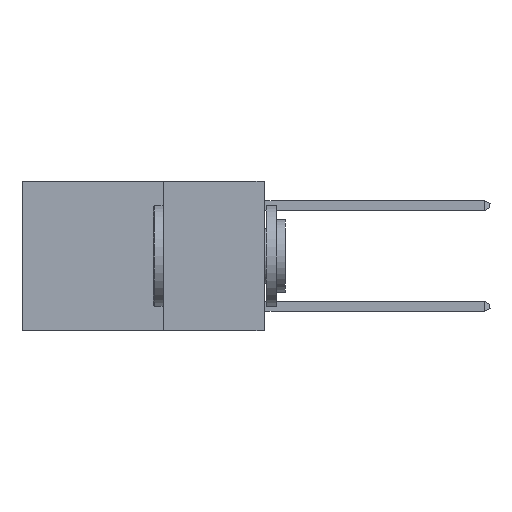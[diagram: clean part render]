
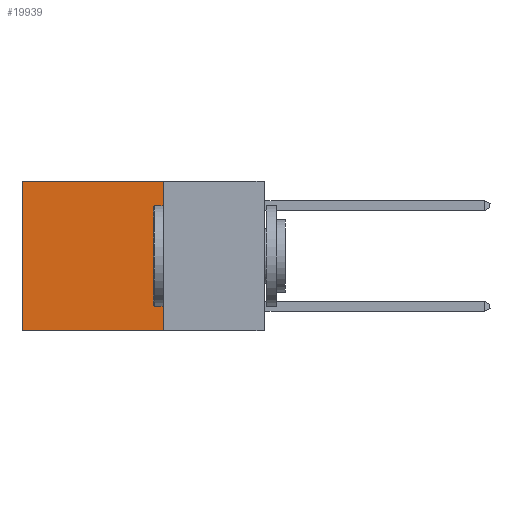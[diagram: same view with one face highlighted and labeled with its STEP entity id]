
A CAD part, left-side view. The second image highlights one B-rep face of the part: STEP entity #19939.
In plain terms, the highlighted planar face has unit normal (-1, 0, 0).
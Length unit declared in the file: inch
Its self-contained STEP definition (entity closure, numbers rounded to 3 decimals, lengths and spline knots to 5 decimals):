
#365 = CARTESIAN_POINT ( 'NONE',  ( 0.2625, 0.6, 0. ) ) ;
#396 = DIRECTION ( 'NONE',  ( 0., 1., 0. ) ) ;
#508 = ORIENTED_EDGE ( 'NONE', *, *, #2461, .F. ) ;
#648 = LINE ( 'NONE', #17903, #14365 ) ;
#1632 = CARTESIAN_POINT ( 'NONE',  ( 0.2625, 0.6, -0.37 ) ) ;
#1991 = DIRECTION ( 'NONE',  ( 1., 0., 0. ) ) ;
#2390 = EDGE_CURVE ( 'NONE', #7936, #6445, #15026, .T. ) ;
#2461 = EDGE_CURVE ( 'NONE', #20029, #6445, #648, .T. ) ;
#2487 = CARTESIAN_POINT ( 'NONE',  ( 0.2625, 0.25, 0. ) ) ;
#4144 = DIRECTION ( 'NONE',  ( 0., 1., 0. ) ) ;
#5660 = EDGE_LOOP ( 'NONE', ( #15953, #508, #22976, #20756 ) ) ;
#5780 = CARTESIAN_POINT ( 'NONE',  ( 0.2625, 0.25, -0.37 ) ) ;
#6138 = PLANE ( 'NONE',  #12309 ) ;
#6346 = LINE ( 'NONE', #7991, #18341 ) ;
#6445 = VERTEX_POINT ( 'NONE', #1632 ) ;
#7911 = FACE_OUTER_BOUND ( 'NONE', #5660, .T. ) ;
#7936 = VERTEX_POINT ( 'NONE', #365 ) ;
#7991 = CARTESIAN_POINT ( 'NONE',  ( 0.2625, 0.25, 0. ) ) ;
#8807 = VECTOR ( 'NONE', #4144, 39.37008 ) ;
#9171 = VERTEX_POINT ( 'NONE', #14637 ) ;
#9235 = DIRECTION ( 'NONE',  ( 0., 0., -1. ) ) ;
#9830 = EDGE_CURVE ( 'NONE', #9171, #7936, #23207, .T. ) ;
#12309 = AXIS2_PLACEMENT_3D ( 'NONE', #13948, #1991, #23422 ) ;
#13948 = CARTESIAN_POINT ( 'NONE',  ( 0.2625, 0.25, 0. ) ) ;
#14033 = DIRECTION ( 'NONE',  ( 0., 0., -1. ) ) ;
#14365 = VECTOR ( 'NONE', #396, 39.37008 ) ;
#14637 = CARTESIAN_POINT ( 'NONE',  ( 0.2625, 0.25, 0. ) ) ;
#15026 = LINE ( 'NONE', #16908, #22020 ) ;
#15953 = ORIENTED_EDGE ( 'NONE', *, *, #2390, .T. ) ;
#16908 = CARTESIAN_POINT ( 'NONE',  ( 0.2625, 0.6, 0. ) ) ;
#17903 = CARTESIAN_POINT ( 'NONE',  ( 0.2625, 0.25, -0.37 ) ) ;
#18341 = VECTOR ( 'NONE', #14033, 39.37008 ) ;
#19939 = ADVANCED_FACE ( 'NONE', ( #7911 ), #6138, .F. ) ;
#20029 = VERTEX_POINT ( 'NONE', #5780 ) ;
#20756 = ORIENTED_EDGE ( 'NONE', *, *, #9830, .T. ) ;
#21745 = EDGE_CURVE ( 'NONE', #9171, #20029, #6346, .T. ) ;
#22020 = VECTOR ( 'NONE', #9235, 39.37008 ) ;
#22976 = ORIENTED_EDGE ( 'NONE', *, *, #21745, .F. ) ;
#23207 = LINE ( 'NONE', #2487, #8807 ) ;
#23422 = DIRECTION ( 'NONE',  ( 0., 0., -1. ) ) ;
